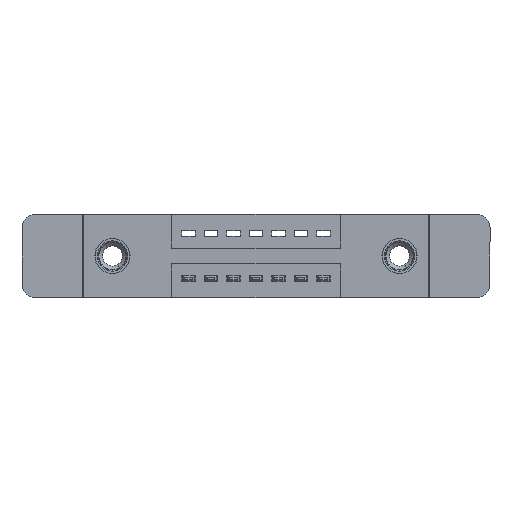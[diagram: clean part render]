
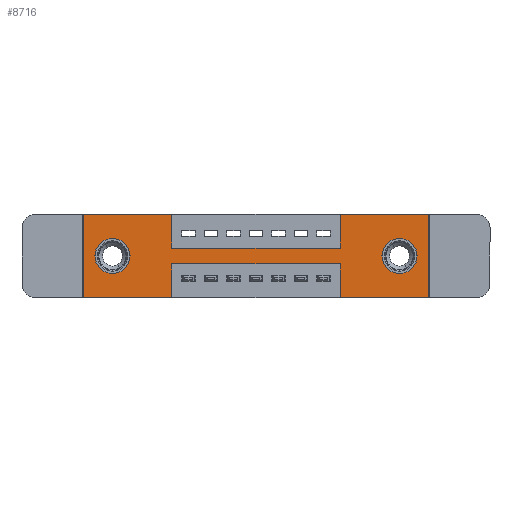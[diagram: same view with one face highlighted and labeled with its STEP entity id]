
A CAD part, front view. The second image highlights one B-rep face of the part: STEP entity #8716.
In plain terms, the highlighted planar face has unit normal (0, -1, 0).
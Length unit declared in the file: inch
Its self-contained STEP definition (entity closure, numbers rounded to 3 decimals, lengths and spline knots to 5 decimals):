
#28 = ORIENTED_EDGE ( 'NONE', *, *, #11690, .F. ) ;
#143 = VECTOR ( 'NONE', #11254, 39.37008 ) ;
#325 = ORIENTED_EDGE ( 'NONE', *, *, #13222, .F. ) ;
#513 = DIRECTION ( 'NONE',  ( 0., 0., -1. ) ) ;
#516 = CARTESIAN_POINT ( 'NONE',  ( 1.535, 0., -0.37 ) ) ;
#600 = CARTESIAN_POINT ( 'NONE',  ( 0.3925, 0., -0.37 ) ) ;
#912 = ORIENTED_EDGE ( 'NONE', *, *, #11424, .F. ) ;
#1175 = CARTESIAN_POINT ( 'NONE',  ( 1.1425, 0., 0. ) ) ;
#1198 = CARTESIAN_POINT ( 'NONE',  ( 0.13, 0., -0.263 ) ) ;
#1366 = VECTOR ( 'NONE', #12086, 39.37008 ) ;
#1616 = LINE ( 'NONE', #11938, #2356 ) ;
#1677 = ORIENTED_EDGE ( 'NONE', *, *, #6913, .F. ) ;
#1697 = AXIS2_PLACEMENT_3D ( 'NONE', #12718, #5858, #3525 ) ;
#1717 = CARTESIAN_POINT ( 'NONE',  ( 0.3925, 0., -0.15 ) ) ;
#1779 = EDGE_CURVE ( 'NONE', #14355, #14883, #5236, .T. ) ;
#1886 = CARTESIAN_POINT ( 'NONE',  ( 1.405, 0., -0.107 ) ) ;
#1894 = CARTESIAN_POINT ( 'NONE',  ( 1.405, 0., -0.185 ) ) ;
#2192 = DIRECTION ( 'NONE',  ( 0., 1., 0. ) ) ;
#2197 = VERTEX_POINT ( 'NONE', #5926 ) ;
#2216 = EDGE_LOOP ( 'NONE', ( #1677, #8621, #912, #4508, #9696, #325, #14674, #6398, #4182, #14053, #12366, #28 ) ) ;
#2320 = VECTOR ( 'NONE', #4153, 39.37008 ) ;
#2356 = VECTOR ( 'NONE', #10133, 39.37008 ) ;
#2374 = DIRECTION ( 'NONE',  ( 0., 0., 1. ) ) ;
#2528 = ORIENTED_EDGE ( 'NONE', *, *, #9761, .T. ) ;
#2566 = VERTEX_POINT ( 'NONE', #7990 ) ;
#2752 = VERTEX_POINT ( 'NONE', #10541 ) ;
#3040 = DIRECTION ( 'NONE',  ( 0., 0., -1. ) ) ;
#3265 = LINE ( 'NONE', #14641, #143 ) ;
#3283 = CARTESIAN_POINT ( 'NONE',  ( 0.13, 0., -0.185 ) ) ;
#3347 = FACE_BOUND ( 'NONE', #7233, .T. ) ;
#3453 = VERTEX_POINT ( 'NONE', #600 ) ;
#3525 = DIRECTION ( 'NONE',  ( 0., 0., -1. ) ) ;
#3596 = CARTESIAN_POINT ( 'NONE',  ( 1.1425, 0., -0.37 ) ) ;
#3797 = VERTEX_POINT ( 'NONE', #1198 ) ;
#3953 = LINE ( 'NONE', #6468, #13503 ) ;
#4020 = DIRECTION ( 'NONE',  ( 0., 1., 0. ) ) ;
#4153 = DIRECTION ( 'NONE',  ( 0., 0., 1. ) ) ;
#4182 = ORIENTED_EDGE ( 'NONE', *, *, #9316, .F. ) ;
#4224 = CARTESIAN_POINT ( 'NONE',  ( 0., 0., -0.37 ) ) ;
#4231 = FACE_OUTER_BOUND ( 'NONE', #2216, .T. ) ;
#4508 = ORIENTED_EDGE ( 'NONE', *, *, #1779, .F. ) ;
#5020 = EDGE_CURVE ( 'NONE', #2197, #14355, #13584, .T. ) ;
#5089 = DIRECTION ( 'NONE',  ( 0., 0., -1. ) ) ;
#5168 = VERTEX_POINT ( 'NONE', #1717 ) ;
#5198 = DIRECTION ( 'NONE',  ( 1., 0., 0. ) ) ;
#5236 = LINE ( 'NONE', #11665, #6320 ) ;
#5287 = ORIENTED_EDGE ( 'NONE', *, *, #13601, .T. ) ;
#5293 = CARTESIAN_POINT ( 'NONE',  ( 0., 0., 0. ) ) ;
#5335 = CARTESIAN_POINT ( 'NONE',  ( 0.3925, 0., 0. ) ) ;
#5589 = CIRCLE ( 'NONE', #12254, 0.078 ) ;
#5663 = EDGE_CURVE ( 'NONE', #11512, #13523, #10826, .T. ) ;
#5804 = VECTOR ( 'NONE', #13675, 39.37008 ) ;
#5858 = DIRECTION ( 'NONE',  ( 0., -1., 0. ) ) ;
#5879 = CARTESIAN_POINT ( 'NONE',  ( 0.3925, 0., 0. ) ) ;
#5926 = CARTESIAN_POINT ( 'NONE',  ( 1.535, 0., 0. ) ) ;
#5958 = DIRECTION ( 'NONE',  ( -1., 0., 0. ) ) ;
#6126 = CARTESIAN_POINT ( 'NONE',  ( 0.3925, 0., -0.37 ) ) ;
#6167 = EDGE_CURVE ( 'NONE', #9712, #2566, #7228, .T. ) ;
#6210 = ORIENTED_EDGE ( 'NONE', *, *, #6167, .T. ) ;
#6320 = VECTOR ( 'NONE', #5958, 39.37008 ) ;
#6379 = VECTOR ( 'NONE', #12189, 39.37008 ) ;
#6398 = ORIENTED_EDGE ( 'NONE', *, *, #12096, .F. ) ;
#6468 = CARTESIAN_POINT ( 'NONE',  ( 0., 0., 0. ) ) ;
#6594 = DIRECTION ( 'NONE',  ( 0., 1., 0. ) ) ;
#6682 = DIRECTION ( 'NONE',  ( 0., 0., 1. ) ) ;
#6744 = LINE ( 'NONE', #7640, #6379 ) ;
#6840 = LINE ( 'NONE', #6126, #1366 ) ;
#6913 = EDGE_CURVE ( 'NONE', #2752, #3453, #6840, .T. ) ;
#6916 = CARTESIAN_POINT ( 'NONE',  ( 0., 0., 0. ) ) ;
#7040 = DIRECTION ( 'NONE',  ( 0., 0., -1. ) ) ;
#7228 = CIRCLE ( 'NONE', #13785, 0.078 ) ;
#7233 = EDGE_LOOP ( 'NONE', ( #5287, #2528 ) ) ;
#7391 = CARTESIAN_POINT ( 'NONE',  ( 1.1425, 0., -0.22 ) ) ;
#7485 = CARTESIAN_POINT ( 'NONE',  ( 1.405, 0., -0.185 ) ) ;
#7493 = VECTOR ( 'NONE', #5089, 39.37008 ) ;
#7620 = CARTESIAN_POINT ( 'NONE',  ( 0., 0., 0. ) ) ;
#7640 = CARTESIAN_POINT ( 'NONE',  ( 1.1425, 0., -0.37 ) ) ;
#7789 = EDGE_LOOP ( 'NONE', ( #6210, #11243 ) ) ;
#7868 = VECTOR ( 'NONE', #8320, 39.37008 ) ;
#7990 = CARTESIAN_POINT ( 'NONE',  ( 1.405, 0., -0.263 ) ) ;
#8038 = PLANE ( 'NONE',  #1697 ) ;
#8230 = LINE ( 'NONE', #14040, #7868 ) ;
#8320 = DIRECTION ( 'NONE',  ( 0., 0., 1. ) ) ;
#8546 = EDGE_CURVE ( 'NONE', #13523, #10255, #13059, .T. ) ;
#8621 = ORIENTED_EDGE ( 'NONE', *, *, #12183, .F. ) ;
#8716 = ADVANCED_FACE ( 'NONE', ( #9151, #3347, #4231 ), #8038, .T. ) ;
#8887 = LINE ( 'NONE', #13559, #5804 ) ;
#9069 = EDGE_CURVE ( 'NONE', #10364, #12833, #8230, .T. ) ;
#9151 = FACE_BOUND ( 'NONE', #7789, .T. ) ;
#9193 = CARTESIAN_POINT ( 'NONE',  ( 0.13, 0., -0.185 ) ) ;
#9316 = EDGE_CURVE ( 'NONE', #10255, #5168, #13619, .T. ) ;
#9555 = CARTESIAN_POINT ( 'NONE',  ( 1.535, 0., 0. ) ) ;
#9696 = ORIENTED_EDGE ( 'NONE', *, *, #5020, .F. ) ;
#9712 = VERTEX_POINT ( 'NONE', #1886 ) ;
#9761 = EDGE_CURVE ( 'NONE', #3797, #12886, #10191, .T. ) ;
#10133 = DIRECTION ( 'NONE',  ( -1., 0., 0. ) ) ;
#10191 = CIRCLE ( 'NONE', #11970, 0.078 ) ;
#10244 = CARTESIAN_POINT ( 'NONE',  ( 0.13, 0., -0.107 ) ) ;
#10255 = VERTEX_POINT ( 'NONE', #5335 ) ;
#10272 = DIRECTION ( 'NONE',  ( 0., 1., 0. ) ) ;
#10364 = VERTEX_POINT ( 'NONE', #12512 ) ;
#10541 = CARTESIAN_POINT ( 'NONE',  ( 0.3925, 0., -0.22 ) ) ;
#10566 = VECTOR ( 'NONE', #7040, 39.37008 ) ;
#10826 = LINE ( 'NONE', #7620, #2320 ) ;
#11243 = ORIENTED_EDGE ( 'NONE', *, *, #11286, .T. ) ;
#11254 = DIRECTION ( 'NONE',  ( 1., 0., 0. ) ) ;
#11286 = EDGE_CURVE ( 'NONE', #2566, #9712, #14295, .T. ) ;
#11304 = VERTEX_POINT ( 'NONE', #7391 ) ;
#11424 = EDGE_CURVE ( 'NONE', #14883, #11304, #6744, .T. ) ;
#11512 = VERTEX_POINT ( 'NONE', #4224 ) ;
#11665 = CARTESIAN_POINT ( 'NONE',  ( 0., 0., -0.37 ) ) ;
#11690 = EDGE_CURVE ( 'NONE', #3453, #11512, #1616, .T. ) ;
#11938 = CARTESIAN_POINT ( 'NONE',  ( 0., 0., -0.37 ) ) ;
#11970 = AXIS2_PLACEMENT_3D ( 'NONE', #3283, #2192, #6682 ) ;
#12086 = DIRECTION ( 'NONE',  ( 0., 0., -1. ) ) ;
#12096 = EDGE_CURVE ( 'NONE', #5168, #10364, #3265, .T. ) ;
#12183 = EDGE_CURVE ( 'NONE', #11304, #2752, #8887, .T. ) ;
#12189 = DIRECTION ( 'NONE',  ( 0., 0., 1. ) ) ;
#12254 = AXIS2_PLACEMENT_3D ( 'NONE', #9193, #10272, #2374 ) ;
#12339 = VECTOR ( 'NONE', #5198, 39.37008 ) ;
#12366 = ORIENTED_EDGE ( 'NONE', *, *, #5663, .F. ) ;
#12512 = CARTESIAN_POINT ( 'NONE',  ( 1.1425, 0., -0.15 ) ) ;
#12718 = CARTESIAN_POINT ( 'NONE',  ( 0., 0., -0.37 ) ) ;
#12833 = VERTEX_POINT ( 'NONE', #1175 ) ;
#12886 = VERTEX_POINT ( 'NONE', #10244 ) ;
#13040 = AXIS2_PLACEMENT_3D ( 'NONE', #7485, #4020, #513 ) ;
#13059 = LINE ( 'NONE', #5293, #12339 ) ;
#13222 = EDGE_CURVE ( 'NONE', #12833, #2197, #3953, .T. ) ;
#13503 = VECTOR ( 'NONE', #14456, 39.37008 ) ;
#13523 = VERTEX_POINT ( 'NONE', #6916 ) ;
#13559 = CARTESIAN_POINT ( 'NONE',  ( 0.3925, 0., -0.22 ) ) ;
#13584 = LINE ( 'NONE', #9555, #7493 ) ;
#13601 = EDGE_CURVE ( 'NONE', #12886, #3797, #5589, .T. ) ;
#13619 = LINE ( 'NONE', #5879, #10566 ) ;
#13675 = DIRECTION ( 'NONE',  ( -1., 0., 0. ) ) ;
#13785 = AXIS2_PLACEMENT_3D ( 'NONE', #1894, #6594, #3040 ) ;
#14040 = CARTESIAN_POINT ( 'NONE',  ( 1.1425, 0., 0. ) ) ;
#14053 = ORIENTED_EDGE ( 'NONE', *, *, #8546, .F. ) ;
#14295 = CIRCLE ( 'NONE', #13040, 0.078 ) ;
#14355 = VERTEX_POINT ( 'NONE', #516 ) ;
#14456 = DIRECTION ( 'NONE',  ( 1., 0., 0. ) ) ;
#14641 = CARTESIAN_POINT ( 'NONE',  ( 0.3925, 0., -0.15 ) ) ;
#14674 = ORIENTED_EDGE ( 'NONE', *, *, #9069, .F. ) ;
#14883 = VERTEX_POINT ( 'NONE', #3596 ) ;
